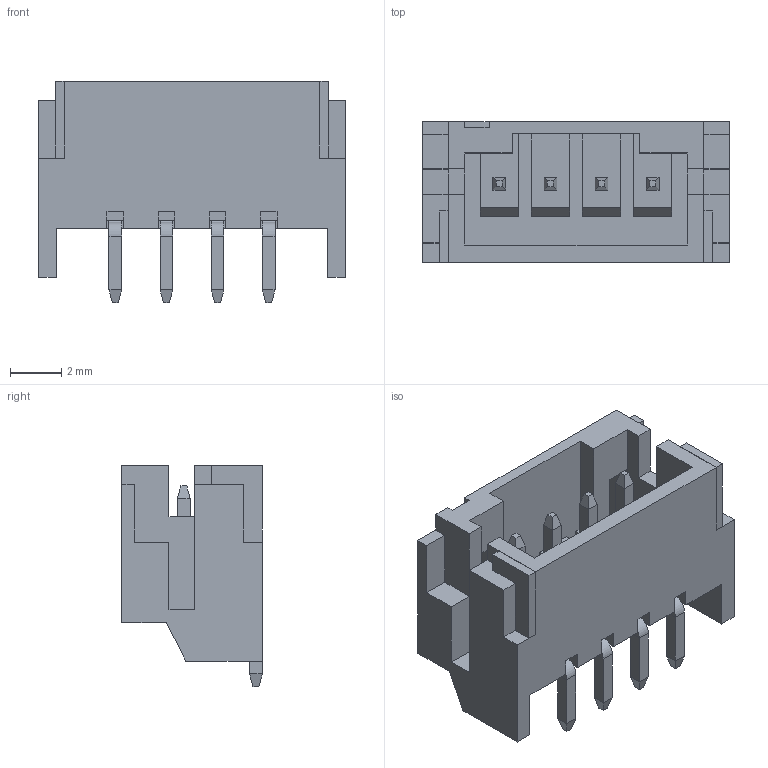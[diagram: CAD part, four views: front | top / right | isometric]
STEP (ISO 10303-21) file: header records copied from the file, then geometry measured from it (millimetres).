
FILE_DESCRIPTION (( 'STEP AP203' ), '1' );
FILE_NAME ('140-504-417-060.STEP', '2020-03-31T20:19:54', ( '' ), ( '' ), 'SwSTEP 2.0', 'SolidWorks 2016', '' );
FILE_SCHEMA (( 'CONFIG_CONTROL_DESIGN' ));
Length unit declared in the file: millimetre
Products named in the file (4): 140-504-417-060; RA SMT Housing_504; RA SMT Contact; RA SMT Pad
Assembly tree (7 placements, depth 2):
  140-504-417-060
    RA SMT Housing_504
    RA SMT Contact  x4
    RA SMT Pad  x2
Bounding box: 12 x 5.5 x 8.65 mm (x, y, z)
Volume: 188.7 mm3; surface area: 675.5 mm2
Topology: 7 solids, 7 shells, 264 faces, 664 edges, 410 vertices
Faces by surface type: plane 248, cylinder 16
Entity records: 5842 total; most frequent: CARTESIAN_POINT 956, ORIENTED_EDGE 944, DIRECTION 836, EDGE_CURVE 472, VECTOR 464, LINE 464, VERTEX_POINT 306, AXIS2_PLACEMENT_3D 186
